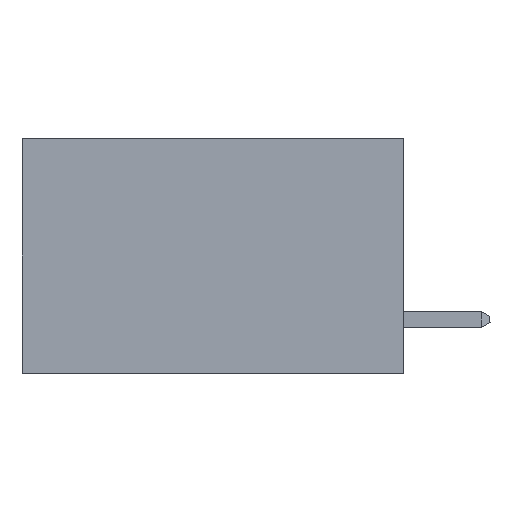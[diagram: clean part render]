
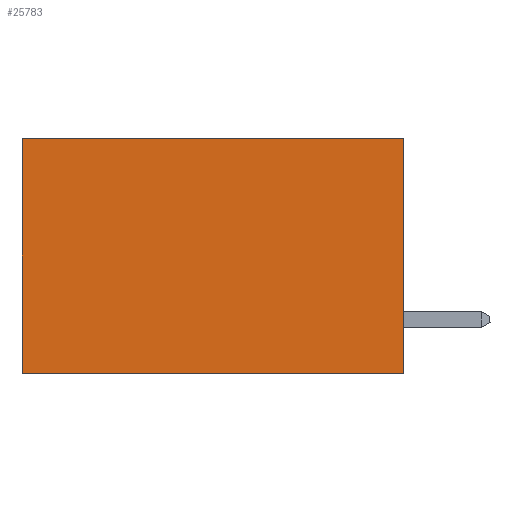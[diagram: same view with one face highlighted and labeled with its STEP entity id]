
A CAD part, left-side view. The second image highlights one B-rep face of the part: STEP entity #25783.
In plain terms, the highlighted planar face has unit normal (-1, 0, 0).
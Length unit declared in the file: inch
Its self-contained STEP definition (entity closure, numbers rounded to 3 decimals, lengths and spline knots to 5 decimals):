
#407 = VERTEX_POINT ( 'NONE', #15458 ) ;
#959 = EDGE_CURVE ( 'NONE', #22024, #9428, #4712, .T. ) ;
#1484 = EDGE_LOOP ( 'NONE', ( #29096, #21576, #28373, #7274 ) ) ;
#1553 = VECTOR ( 'NONE', #7262, 39.37008 ) ;
#2198 = VERTEX_POINT ( 'NONE', #10363 ) ;
#3532 = LINE ( 'NONE', #19063, #38506 ) ;
#4712 = LINE ( 'NONE', #9152, #33771 ) ;
#6915 = AXIS2_PLACEMENT_3D ( 'NONE', #25840, #28913, #10983 ) ;
#7262 = DIRECTION ( 'NONE',  ( 0., 0., -1. ) ) ;
#7274 = ORIENTED_EDGE ( 'NONE', *, *, #28199, .T. ) ;
#8453 = EDGE_CURVE ( 'NONE', #2198, #9428, #3532, .T. ) ;
#8887 = CARTESIAN_POINT ( 'NONE',  ( 0.2875, 0.6, -0.37 ) ) ;
#9152 = CARTESIAN_POINT ( 'NONE',  ( 0.2875, 0.6, 0. ) ) ;
#9428 = VERTEX_POINT ( 'NONE', #8887 ) ;
#10263 = LINE ( 'NONE', #11931, #34018 ) ;
#10363 = CARTESIAN_POINT ( 'NONE',  ( 0.2875, 0., -0.37 ) ) ;
#10983 = DIRECTION ( 'NONE',  ( 0., 0., -1. ) ) ;
#11931 = CARTESIAN_POINT ( 'NONE',  ( 0.2875, 0., 0. ) ) ;
#15150 = FACE_OUTER_BOUND ( 'NONE', #1484, .T. ) ;
#15458 = CARTESIAN_POINT ( 'NONE',  ( 0.2875, 0., 0. ) ) ;
#19063 = CARTESIAN_POINT ( 'NONE',  ( 0.2875, 0., -0.37 ) ) ;
#21135 = DIRECTION ( 'NONE',  ( 0., 0., -1. ) ) ;
#21576 = ORIENTED_EDGE ( 'NONE', *, *, #8453, .F. ) ;
#22024 = VERTEX_POINT ( 'NONE', #31628 ) ;
#22082 = DIRECTION ( 'NONE',  ( 0., 1., 0. ) ) ;
#22951 = PLANE ( 'NONE',  #6915 ) ;
#25763 = LINE ( 'NONE', #31224, #1553 ) ;
#25783 = ADVANCED_FACE ( 'NONE', ( #15150 ), #22951, .F. ) ;
#25840 = CARTESIAN_POINT ( 'NONE',  ( 0.2875, 0., 0. ) ) ;
#28199 = EDGE_CURVE ( 'NONE', #407, #22024, #10263, .T. ) ;
#28373 = ORIENTED_EDGE ( 'NONE', *, *, #28402, .F. ) ;
#28402 = EDGE_CURVE ( 'NONE', #407, #2198, #25763, .T. ) ;
#28913 = DIRECTION ( 'NONE',  ( 1., 0., 0. ) ) ;
#29096 = ORIENTED_EDGE ( 'NONE', *, *, #959, .T. ) ;
#31224 = CARTESIAN_POINT ( 'NONE',  ( 0.2875, 0., 0. ) ) ;
#31628 = CARTESIAN_POINT ( 'NONE',  ( 0.2875, 0.6, 0. ) ) ;
#32756 = DIRECTION ( 'NONE',  ( 0., 1., 0. ) ) ;
#33771 = VECTOR ( 'NONE', #21135, 39.37008 ) ;
#34018 = VECTOR ( 'NONE', #32756, 39.37008 ) ;
#38506 = VECTOR ( 'NONE', #22082, 39.37008 ) ;
